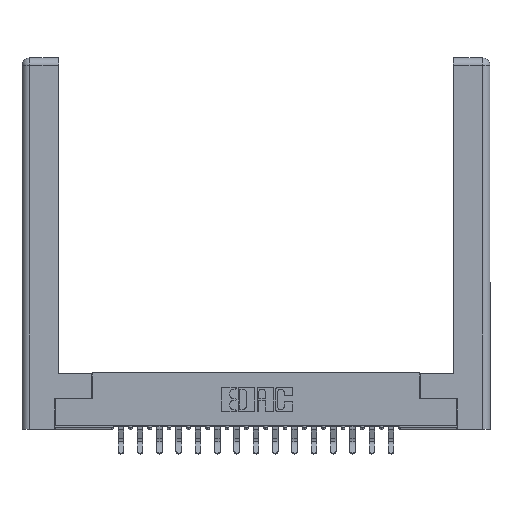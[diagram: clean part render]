
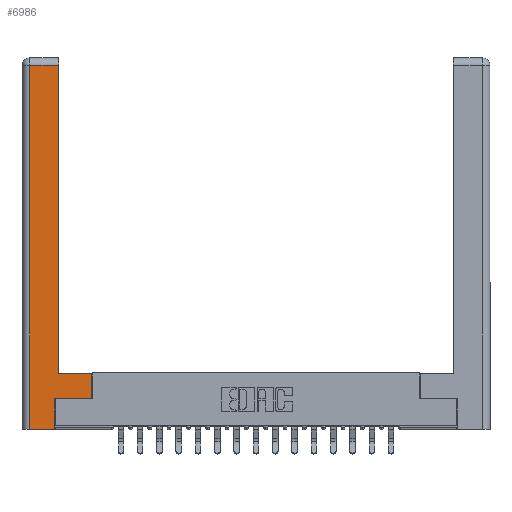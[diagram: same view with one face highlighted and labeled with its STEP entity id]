
A CAD part, top view. The second image highlights one B-rep face of the part: STEP entity #6986.
In plain terms, the highlighted planar face has unit normal (0, 0, 1).
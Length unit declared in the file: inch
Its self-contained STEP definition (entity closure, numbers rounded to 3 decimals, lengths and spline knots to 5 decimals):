
#187 = EDGE_CURVE ( 'NONE', #561, #6891, #21814, .T. ) ;
#464 = ORIENTED_EDGE ( 'NONE', *, *, #5057, .T. ) ;
#561 = VERTEX_POINT ( 'NONE', #9840 ) ;
#573 = VERTEX_POINT ( 'NONE', #20032 ) ;
#1576 = CARTESIAN_POINT ( 'NONE',  ( 0.565, 0.245, 0. ) ) ;
#1623 = EDGE_CURVE ( 'NONE', #573, #21207, #2282, .T. ) ;
#2282 = LINE ( 'NONE', #22009, #17984 ) ;
#2502 = EDGE_CURVE ( 'NONE', #13007, #573, #10331, .T. ) ;
#2812 = DIRECTION ( 'NONE',  ( 0., 1., 0. ) ) ;
#2947 = VERTEX_POINT ( 'NONE', #14546 ) ;
#3930 = CARTESIAN_POINT ( 'NONE',  ( 0., 0., 0. ) ) ;
#4162 = DIRECTION ( 'NONE',  ( 0., 0., -1. ) ) ;
#4218 = ORIENTED_EDGE ( 'NONE', *, *, #2502, .T. ) ;
#4314 = EDGE_CURVE ( 'NONE', #6891, #2947, #21807, .T. ) ;
#4483 = VECTOR ( 'NONE', #16426, 39.37008 ) ;
#4488 = LINE ( 'NONE', #8662, #11257 ) ;
#4964 = DIRECTION ( 'NONE',  ( 0., -1., 0. ) ) ;
#4970 = LINE ( 'NONE', #11813, #6052 ) ;
#5057 = EDGE_CURVE ( 'NONE', #2947, #18701, #4488, .T. ) ;
#5357 = DIRECTION ( 'NONE',  ( 1., 0., 0. ) ) ;
#5386 = ORIENTED_EDGE ( 'NONE', *, *, #187, .T. ) ;
#6052 = VECTOR ( 'NONE', #19916, 39.37008 ) ;
#6137 = CARTESIAN_POINT ( 'NONE',  ( 0.0615, 0., 0. ) ) ;
#6769 = VERTEX_POINT ( 'NONE', #6799 ) ;
#6799 = CARTESIAN_POINT ( 'NONE',  ( 0.565, 0.245, 0. ) ) ;
#6859 = CARTESIAN_POINT ( 'NONE',  ( 0.295, 2.94, 0. ) ) ;
#6891 = VERTEX_POINT ( 'NONE', #6137 ) ;
#6986 = ADVANCED_FACE ( 'NONE', ( #12805 ), #21392, .F. ) ;
#7669 = AXIS2_PLACEMENT_3D ( 'NONE', #3930, #4162, #12145 ) ;
#8662 = CARTESIAN_POINT ( 'NONE',  ( 0.265, 0.245, 0. ) ) ;
#8924 = CARTESIAN_POINT ( 'NONE',  ( 0.265, 0.245, 0. ) ) ;
#9840 = CARTESIAN_POINT ( 'NONE',  ( 0.0615, 2.94, 0. ) ) ;
#10051 = CARTESIAN_POINT ( 'NONE',  ( 0.295, 0.45, 0. ) ) ;
#10331 = LINE ( 'NONE', #10051, #12552 ) ;
#11257 = VECTOR ( 'NONE', #13860, 39.37008 ) ;
#11433 = ORIENTED_EDGE ( 'NONE', *, *, #1623, .T. ) ;
#11520 = DIRECTION ( 'NONE',  ( 0., 1., 0. ) ) ;
#11572 = ORIENTED_EDGE ( 'NONE', *, *, #19749, .T. ) ;
#11729 = ORIENTED_EDGE ( 'NONE', *, *, #4314, .T. ) ;
#11813 = CARTESIAN_POINT ( 'NONE',  ( 0.0615, 2.94, 0. ) ) ;
#12144 = EDGE_CURVE ( 'NONE', #21207, #561, #4970, .T. ) ;
#12145 = DIRECTION ( 'NONE',  ( -1., 0., 0. ) ) ;
#12552 = VECTOR ( 'NONE', #13715, 39.37008 ) ;
#12701 = LINE ( 'NONE', #1576, #17848 ) ;
#12800 = CARTESIAN_POINT ( 'NONE',  ( 0.265, 0., 0. ) ) ;
#12805 = FACE_OUTER_BOUND ( 'NONE', #20667, .T. ) ;
#13007 = VERTEX_POINT ( 'NONE', #17884 ) ;
#13715 = DIRECTION ( 'NONE',  ( -1., 0., 0. ) ) ;
#13860 = DIRECTION ( 'NONE',  ( 0., 1., 0. ) ) ;
#14546 = CARTESIAN_POINT ( 'NONE',  ( 0.265, 0., 0. ) ) ;
#14825 = EDGE_CURVE ( 'NONE', #6769, #13007, #17901, .T. ) ;
#16426 = DIRECTION ( 'NONE',  ( 1., 0., 0. ) ) ;
#17547 = ORIENTED_EDGE ( 'NONE', *, *, #14825, .T. ) ;
#17848 = VECTOR ( 'NONE', #5357, 39.37008 ) ;
#17884 = CARTESIAN_POINT ( 'NONE',  ( 0.565, 0.45, 0. ) ) ;
#17901 = LINE ( 'NONE', #21753, #21397 ) ;
#17984 = VECTOR ( 'NONE', #2812, 39.37008 ) ;
#18701 = VERTEX_POINT ( 'NONE', #8924 ) ;
#19749 = EDGE_CURVE ( 'NONE', #18701, #6769, #12701, .T. ) ;
#19916 = DIRECTION ( 'NONE',  ( -1., 0., 0. ) ) ;
#20032 = CARTESIAN_POINT ( 'NONE',  ( 0.295, 0.45, 0. ) ) ;
#20482 = CARTESIAN_POINT ( 'NONE',  ( 0.0615, 0., 0. ) ) ;
#20667 = EDGE_LOOP ( 'NONE', ( #11433, #21711, #5386, #11729, #464, #11572, #17547, #4218 ) ) ;
#21207 = VERTEX_POINT ( 'NONE', #6859 ) ;
#21276 = VECTOR ( 'NONE', #4964, 39.37008 ) ;
#21392 = PLANE ( 'NONE',  #7669 ) ;
#21397 = VECTOR ( 'NONE', #11520, 39.37008 ) ;
#21711 = ORIENTED_EDGE ( 'NONE', *, *, #12144, .T. ) ;
#21753 = CARTESIAN_POINT ( 'NONE',  ( 0.565, 0.45, 0. ) ) ;
#21807 = LINE ( 'NONE', #12800, #4483 ) ;
#21814 = LINE ( 'NONE', #20482, #21276 ) ;
#22009 = CARTESIAN_POINT ( 'NONE',  ( 0.295, 3., 0. ) ) ;
